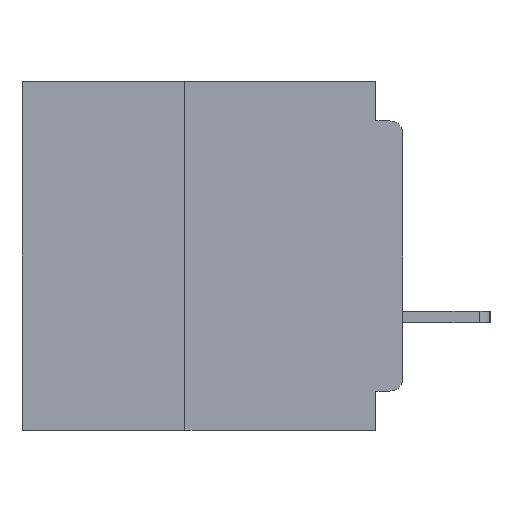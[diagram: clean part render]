
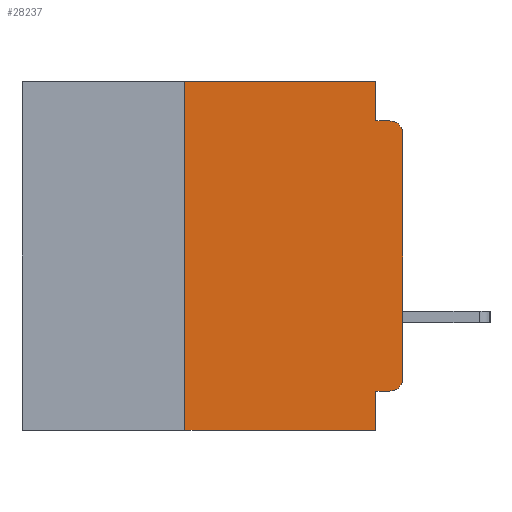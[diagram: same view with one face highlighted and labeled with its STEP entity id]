
A CAD part, left-side view. The second image highlights one B-rep face of the part: STEP entity #28237.
In plain terms, the highlighted planar face has unit normal (-1, 0, 0).
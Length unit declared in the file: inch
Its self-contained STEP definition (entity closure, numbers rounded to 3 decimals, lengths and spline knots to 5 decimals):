
#35 = CARTESIAN_POINT ( 'NONE',  ( 0., 0.015, -0.06 ) ) ;
#53 = CARTESIAN_POINT ( 'NONE',  ( 0., 0., -0.06 ) ) ;
#450 = EDGE_CURVE ( 'NONE', #793, #31352, #42198, .T. ) ;
#793 = VERTEX_POINT ( 'NONE', #10052 ) ;
#2257 = AXIS2_PLACEMENT_3D ( 'NONE', #35, #28145, #4096 ) ;
#2270 = EDGE_CURVE ( 'NONE', #28959, #49504, #6261, .T. ) ;
#3440 = VERTEX_POINT ( 'NONE', #37908 ) ;
#3550 = VECTOR ( 'NONE', #44665, 39.37008 ) ;
#4096 = DIRECTION ( 'NONE',  ( 0., 0., -1. ) ) ;
#4228 = DIRECTION ( 'NONE',  ( 0., 0., -1. ) ) ;
#4313 = CARTESIAN_POINT ( 'NONE',  ( 0., 0., -0.045 ) ) ;
#4506 = ORIENTED_EDGE ( 'NONE', *, *, #11742, .T. ) ;
#5723 = EDGE_CURVE ( 'NONE', #49504, #35194, #36487, .T. ) ;
#5763 = CARTESIAN_POINT ( 'NONE',  ( 0., 0.031, -0.4 ) ) ;
#6261 = LINE ( 'NONE', #43081, #16967 ) ;
#6970 = ORIENTED_EDGE ( 'NONE', *, *, #50493, .T. ) ;
#7193 = ORIENTED_EDGE ( 'NONE', *, *, #23557, .T. ) ;
#8977 = LINE ( 'NONE', #32278, #29055 ) ;
#9082 = DIRECTION ( 'NONE',  ( 0., 0., -1. ) ) ;
#10033 = CARTESIAN_POINT ( 'NONE',  ( 0., 0.031, 0. ) ) ;
#10052 = CARTESIAN_POINT ( 'NONE',  ( 0., 0.015, -0.355 ) ) ;
#10076 = DIRECTION ( 'NONE',  ( -1., 0., 0. ) ) ;
#11742 = EDGE_CURVE ( 'NONE', #3440, #42655, #19966, .T. ) ;
#12375 = CIRCLE ( 'NONE', #2257, 0.015 ) ;
#14183 = DIRECTION ( 'NONE',  ( 0., 0., 1. ) ) ;
#14875 = CARTESIAN_POINT ( 'NONE',  ( 0., 0.031, -0.045 ) ) ;
#15821 = ORIENTED_EDGE ( 'NONE', *, *, #40965, .F. ) ;
#15904 = EDGE_CURVE ( 'NONE', #31251, #28959, #25188, .T. ) ;
#16908 = DIRECTION ( 'NONE',  ( 0., 0., -1. ) ) ;
#16967 = VECTOR ( 'NONE', #43299, 39.37008 ) ;
#17504 = AXIS2_PLACEMENT_3D ( 'NONE', #32836, #40873, #16908 ) ;
#19966 = LINE ( 'NONE', #49953, #28093 ) ;
#19969 = ORIENTED_EDGE ( 'NONE', *, *, #35373, .T. ) ;
#20718 = ORIENTED_EDGE ( 'NONE', *, *, #15904, .F. ) ;
#20749 = FACE_OUTER_BOUND ( 'NONE', #44357, .T. ) ;
#21034 = CARTESIAN_POINT ( 'NONE',  ( 0., 0.25, -0.4 ) ) ;
#21266 = LINE ( 'NONE', #4313, #42502 ) ;
#22041 = EDGE_CURVE ( 'NONE', #35194, #28551, #21266, .T. ) ;
#23557 = EDGE_CURVE ( 'NONE', #793, #3440, #46077, .T. ) ;
#25048 = DIRECTION ( 'NONE',  ( 0., 0., 1. ) ) ;
#25188 = LINE ( 'NONE', #21034, #45102 ) ;
#28093 = VECTOR ( 'NONE', #14183, 39.37008 ) ;
#28145 = DIRECTION ( 'NONE',  ( -1., 0., 0. ) ) ;
#28237 = ADVANCED_FACE ( 'NONE', ( #20749 ), #36849, .F. ) ;
#28551 = VERTEX_POINT ( 'NONE', #31293 ) ;
#28959 = VERTEX_POINT ( 'NONE', #37836 ) ;
#29055 = VECTOR ( 'NONE', #4228, 39.37008 ) ;
#30515 = ORIENTED_EDGE ( 'NONE', *, *, #22041, .F. ) ;
#31251 = VERTEX_POINT ( 'NONE', #48620 ) ;
#31293 = CARTESIAN_POINT ( 'NONE',  ( 0., 0.015, -0.045 ) ) ;
#31352 = VERTEX_POINT ( 'NONE', #37687 ) ;
#31768 = AXIS2_PLACEMENT_3D ( 'NONE', #34037, #10076, #38052 ) ;
#32278 = CARTESIAN_POINT ( 'NONE',  ( 0., 0.031, -0.4 ) ) ;
#32362 = DIRECTION ( 'NONE',  ( 0., -1., 0. ) ) ;
#32836 = CARTESIAN_POINT ( 'NONE',  ( 0., 0.437, 0. ) ) ;
#33266 = CARTESIAN_POINT ( 'NONE',  ( 0., 0.031, 0. ) ) ;
#34037 = CARTESIAN_POINT ( 'NONE',  ( 0., 0.015, -0.34 ) ) ;
#35194 = VERTEX_POINT ( 'NONE', #14875 ) ;
#35242 = VECTOR ( 'NONE', #9082, 39.37008 ) ;
#35373 = EDGE_CURVE ( 'NONE', #42655, #28551, #12375, .T. ) ;
#35455 = ORIENTED_EDGE ( 'NONE', *, *, #2270, .F. ) ;
#35552 = LINE ( 'NONE', #40733, #3550 ) ;
#36487 = LINE ( 'NONE', #33266, #35242 ) ;
#36849 = PLANE ( 'NONE',  #17504 ) ;
#37687 = CARTESIAN_POINT ( 'NONE',  ( 0., 0.031, -0.355 ) ) ;
#37836 = CARTESIAN_POINT ( 'NONE',  ( 0., 0.25, 0. ) ) ;
#37908 = CARTESIAN_POINT ( 'NONE',  ( 0., 0., -0.34 ) ) ;
#38052 = DIRECTION ( 'NONE',  ( 0., 0., -1. ) ) ;
#39421 = VERTEX_POINT ( 'NONE', #5763 ) ;
#40733 = CARTESIAN_POINT ( 'NONE',  ( 0., 0.437, -0.4 ) ) ;
#40873 = DIRECTION ( 'NONE',  ( 1., 0., 0. ) ) ;
#40965 = EDGE_CURVE ( 'NONE', #31352, #39421, #8977, .T. ) ;
#42057 = CARTESIAN_POINT ( 'NONE',  ( 0., 0., -0.355 ) ) ;
#42198 = LINE ( 'NONE', #42057, #51320 ) ;
#42502 = VECTOR ( 'NONE', #32362, 39.37008 ) ;
#42573 = DIRECTION ( 'NONE',  ( 0., 1., 0. ) ) ;
#42655 = VERTEX_POINT ( 'NONE', #53 ) ;
#43081 = CARTESIAN_POINT ( 'NONE',  ( 0., 0.437, 0. ) ) ;
#43299 = DIRECTION ( 'NONE',  ( 0., -1., 0. ) ) ;
#43863 = ORIENTED_EDGE ( 'NONE', *, *, #5723, .F. ) ;
#44357 = EDGE_LOOP ( 'NONE', ( #4506, #19969, #30515, #43863, #35455, #20718, #6970, #15821, #50135, #7193 ) ) ;
#44665 = DIRECTION ( 'NONE',  ( 0., -1., 0. ) ) ;
#45102 = VECTOR ( 'NONE', #25048, 39.37008 ) ;
#46077 = CIRCLE ( 'NONE', #31768, 0.015 ) ;
#48620 = CARTESIAN_POINT ( 'NONE',  ( 0., 0.25, -0.4 ) ) ;
#49504 = VERTEX_POINT ( 'NONE', #10033 ) ;
#49953 = CARTESIAN_POINT ( 'NONE',  ( 0., 0., 0. ) ) ;
#50135 = ORIENTED_EDGE ( 'NONE', *, *, #450, .F. ) ;
#50493 = EDGE_CURVE ( 'NONE', #31251, #39421, #35552, .T. ) ;
#51320 = VECTOR ( 'NONE', #42573, 39.37008 ) ;
